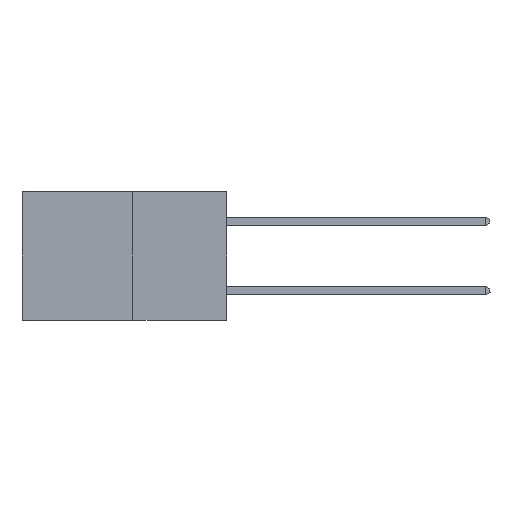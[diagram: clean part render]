
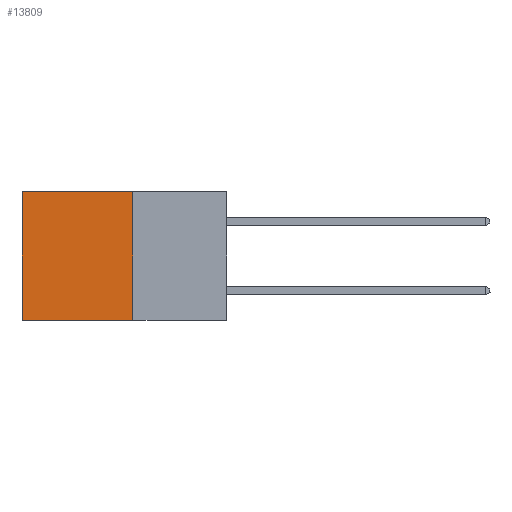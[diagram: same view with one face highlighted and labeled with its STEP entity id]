
A CAD part, left-side view. The second image highlights one B-rep face of the part: STEP entity #13809.
In plain terms, the highlighted planar face has unit normal (-1, 0, 0).
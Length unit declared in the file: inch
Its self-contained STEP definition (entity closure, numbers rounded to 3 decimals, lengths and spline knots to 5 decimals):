
#1474 = CARTESIAN_POINT ( 'NONE',  ( 0.277, 0.27, -0.37 ) ) ;
#2562 = CARTESIAN_POINT ( 'NONE',  ( 0.277, 0.59, 0. ) ) ;
#3080 = VECTOR ( 'NONE', #10015, 39.37008 ) ;
#4370 = VERTEX_POINT ( 'NONE', #5272 ) ;
#5074 = VERTEX_POINT ( 'NONE', #1474 ) ;
#5272 = CARTESIAN_POINT ( 'NONE',  ( 0.277, 0.59, -0.37 ) ) ;
#5498 = CARTESIAN_POINT ( 'NONE',  ( 0.277, 0.27, 0. ) ) ;
#6007 = VERTEX_POINT ( 'NONE', #2562 ) ;
#7046 = VECTOR ( 'NONE', #19686, 39.37008 ) ;
#7150 = DIRECTION ( 'NONE',  ( 0., 0., -1. ) ) ;
#7360 = DIRECTION ( 'NONE',  ( 0., 0., -1. ) ) ;
#7753 = ORIENTED_EDGE ( 'NONE', *, *, #16703, .T. ) ;
#7962 = AXIS2_PLACEMENT_3D ( 'NONE', #10244, #16667, #7150 ) ;
#8460 = CARTESIAN_POINT ( 'NONE',  ( 0.277, 0.27, -0.37 ) ) ;
#8684 = VECTOR ( 'NONE', #19471, 39.37008 ) ;
#10015 = DIRECTION ( 'NONE',  ( 0., 0., -1. ) ) ;
#10244 = CARTESIAN_POINT ( 'NONE',  ( 0.277, 0.27, -0.37 ) ) ;
#10600 = FACE_OUTER_BOUND ( 'NONE', #14292, .T. ) ;
#11546 = CARTESIAN_POINT ( 'NONE',  ( 0.277, 0.27, 0. ) ) ;
#11724 = LINE ( 'NONE', #5498, #7046 ) ;
#11836 = PLANE ( 'NONE',  #7962 ) ;
#12376 = EDGE_CURVE ( 'NONE', #15929, #5074, #16003, .T. ) ;
#12429 = ORIENTED_EDGE ( 'NONE', *, *, #12376, .F. ) ;
#12439 = LINE ( 'NONE', #8460, #8684 ) ;
#13583 = VECTOR ( 'NONE', #7360, 39.37008 ) ;
#13809 = ADVANCED_FACE ( 'NONE', ( #10600 ), #11836, .F. ) ;
#14174 = ORIENTED_EDGE ( 'NONE', *, *, #15473, .T. ) ;
#14292 = EDGE_LOOP ( 'NONE', ( #14174, #19868, #12429, #7753 ) ) ;
#14795 = CARTESIAN_POINT ( 'NONE',  ( 0.277, 0.27, -0.37 ) ) ;
#15473 = EDGE_CURVE ( 'NONE', #6007, #4370, #17263, .T. ) ;
#15929 = VERTEX_POINT ( 'NONE', #11546 ) ;
#16003 = LINE ( 'NONE', #14795, #3080 ) ;
#16667 = DIRECTION ( 'NONE',  ( 1., 0., 0. ) ) ;
#16703 = EDGE_CURVE ( 'NONE', #15929, #6007, #11724, .T. ) ;
#17263 = LINE ( 'NONE', #18396, #13583 ) ;
#18396 = CARTESIAN_POINT ( 'NONE',  ( 0.277, 0.59, -0.37 ) ) ;
#19471 = DIRECTION ( 'NONE',  ( 0., 1., 0. ) ) ;
#19686 = DIRECTION ( 'NONE',  ( 0., 1., 0. ) ) ;
#19768 = EDGE_CURVE ( 'NONE', #5074, #4370, #12439, .T. ) ;
#19868 = ORIENTED_EDGE ( 'NONE', *, *, #19768, .F. ) ;
